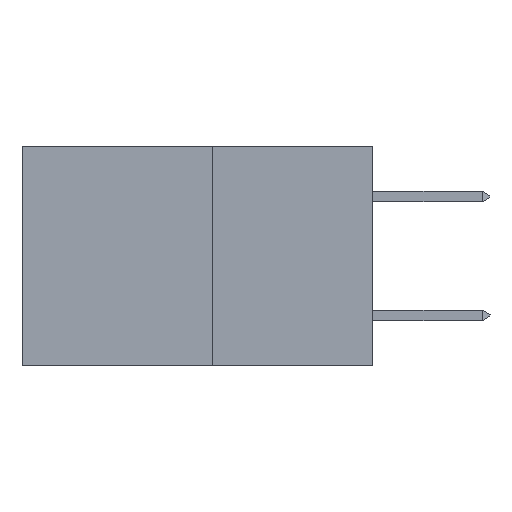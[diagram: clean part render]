
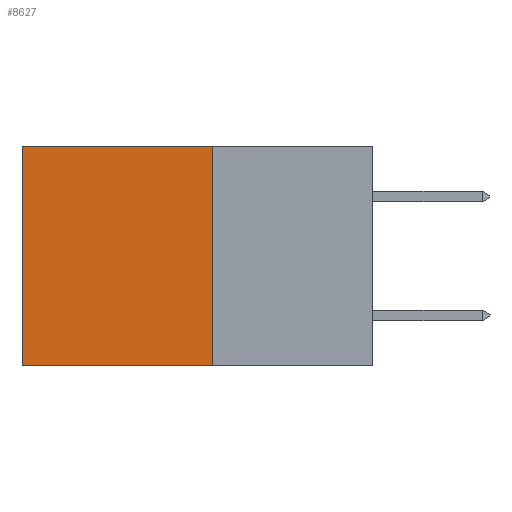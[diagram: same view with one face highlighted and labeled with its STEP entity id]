
A CAD part, left-side view. The second image highlights one B-rep face of the part: STEP entity #8627.
In plain terms, the highlighted planar face has unit normal (-1, 0, 0).
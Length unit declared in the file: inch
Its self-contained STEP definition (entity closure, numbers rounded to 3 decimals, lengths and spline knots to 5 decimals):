
#1155 = LINE ( 'NONE', #14823, #19332 ) ;
#2344 = DIRECTION ( 'NONE',  ( 0., 0., -1. ) ) ;
#3654 = DIRECTION ( 'NONE',  ( 0., 0., -1. ) ) ;
#4110 = ORIENTED_EDGE ( 'NONE', *, *, #4503, .F. ) ;
#4258 = FACE_OUTER_BOUND ( 'NONE', #21831, .T. ) ;
#4503 = EDGE_CURVE ( 'NONE', #5758, #20515, #17288, .T. ) ;
#5758 = VERTEX_POINT ( 'NONE', #11561 ) ;
#5820 = CARTESIAN_POINT ( 'NONE',  ( 0.277, 0.27, 0. ) ) ;
#6069 = EDGE_CURVE ( 'NONE', #20515, #16563, #13760, .T. ) ;
#6678 = AXIS2_PLACEMENT_3D ( 'NONE', #9588, #13224, #2344 ) ;
#6932 = CARTESIAN_POINT ( 'NONE',  ( 0.277, 0.59, -0.37 ) ) ;
#8627 = ADVANCED_FACE ( 'NONE', ( #4258 ), #11396, .F. ) ;
#9588 = CARTESIAN_POINT ( 'NONE',  ( 0.277, 0.27, -0.37 ) ) ;
#10559 = ORIENTED_EDGE ( 'NONE', *, *, #6069, .F. ) ;
#11396 = PLANE ( 'NONE',  #6678 ) ;
#11561 = CARTESIAN_POINT ( 'NONE',  ( 0.277, 0.27, 0. ) ) ;
#12069 = ORIENTED_EDGE ( 'NONE', *, *, #21633, .T. ) ;
#12355 = CARTESIAN_POINT ( 'NONE',  ( 0.277, 0.27, -0.37 ) ) ;
#12448 = VECTOR ( 'NONE', #3654, 39.37008 ) ;
#12706 = CARTESIAN_POINT ( 'NONE',  ( 0.277, 0.27, -0.37 ) ) ;
#13224 = DIRECTION ( 'NONE',  ( 1., 0., 0. ) ) ;
#13760 = LINE ( 'NONE', #12355, #22827 ) ;
#13777 = LINE ( 'NONE', #5820, #23411 ) ;
#14180 = DIRECTION ( 'NONE',  ( 0., 1., 0. ) ) ;
#14823 = CARTESIAN_POINT ( 'NONE',  ( 0.277, 0.59, -0.37 ) ) ;
#16140 = EDGE_CURVE ( 'NONE', #5758, #17642, #13777, .T. ) ;
#16563 = VERTEX_POINT ( 'NONE', #6932 ) ;
#17288 = LINE ( 'NONE', #12706, #12448 ) ;
#17642 = VERTEX_POINT ( 'NONE', #20679 ) ;
#18512 = DIRECTION ( 'NONE',  ( 0., 1., 0. ) ) ;
#19302 = ORIENTED_EDGE ( 'NONE', *, *, #16140, .T. ) ;
#19332 = VECTOR ( 'NONE', #22104, 39.37008 ) ;
#19933 = CARTESIAN_POINT ( 'NONE',  ( 0.277, 0.27, -0.37 ) ) ;
#20515 = VERTEX_POINT ( 'NONE', #19933 ) ;
#20679 = CARTESIAN_POINT ( 'NONE',  ( 0.277, 0.59, 0. ) ) ;
#21633 = EDGE_CURVE ( 'NONE', #17642, #16563, #1155, .T. ) ;
#21831 = EDGE_LOOP ( 'NONE', ( #12069, #10559, #4110, #19302 ) ) ;
#22104 = DIRECTION ( 'NONE',  ( 0., 0., -1. ) ) ;
#22827 = VECTOR ( 'NONE', #14180, 39.37008 ) ;
#23411 = VECTOR ( 'NONE', #18512, 39.37008 ) ;
